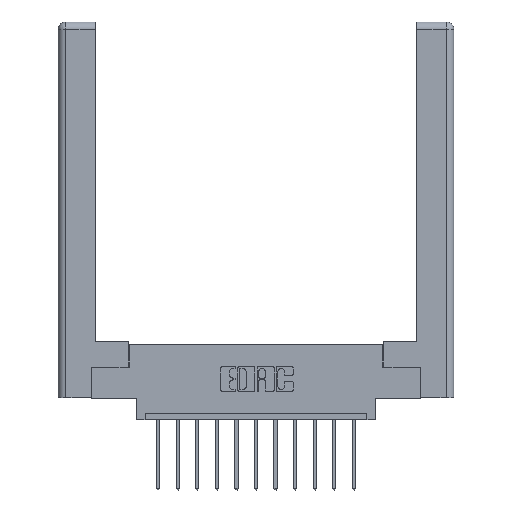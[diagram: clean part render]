
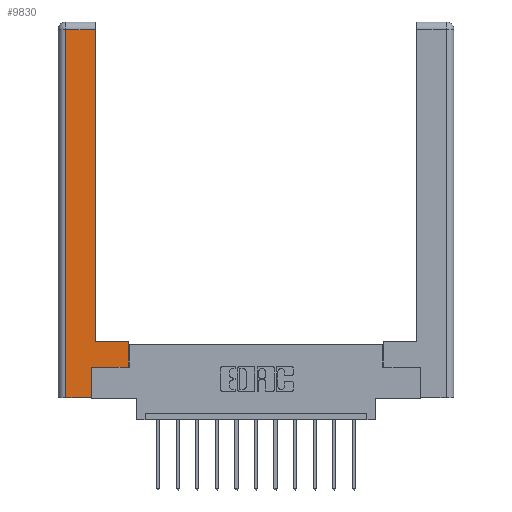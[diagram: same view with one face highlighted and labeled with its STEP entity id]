
A CAD part, top view. The second image highlights one B-rep face of the part: STEP entity #9830.
In plain terms, the highlighted planar face has unit normal (0, 0, 1).
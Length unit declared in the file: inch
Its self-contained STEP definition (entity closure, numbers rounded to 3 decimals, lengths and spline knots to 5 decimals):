
#42 = ORIENTED_EDGE ( 'NONE', *, *, #12930, .T. ) ;
#120 = ORIENTED_EDGE ( 'NONE', *, *, #3742, .T. ) ;
#943 = EDGE_LOOP ( 'NONE', ( #3057, #42, #7764, #14401, #6972, #7880, #6379, #120 ) ) ;
#1010 = CARTESIAN_POINT ( 'NONE',  ( 0., 0., 0. ) ) ;
#1068 = DIRECTION ( 'NONE',  ( -1., 0., 0. ) ) ;
#1400 = EDGE_CURVE ( 'NONE', #2829, #3578, #2583, .T. ) ;
#1668 = VECTOR ( 'NONE', #1682, 39.37008 ) ;
#1682 = DIRECTION ( 'NONE',  ( 0., 1., 0. ) ) ;
#1726 = CARTESIAN_POINT ( 'NONE',  ( 0.295, 0.45, 0. ) ) ;
#2386 = CARTESIAN_POINT ( 'NONE',  ( 0.295, 2.94, 0. ) ) ;
#2583 = LINE ( 'NONE', #3618, #6916 ) ;
#2677 = FACE_OUTER_BOUND ( 'NONE', #943, .T. ) ;
#2763 = DIRECTION ( 'NONE',  ( 1., 0., 0. ) ) ;
#2829 = VERTEX_POINT ( 'NONE', #6642 ) ;
#2945 = EDGE_CURVE ( 'NONE', #5916, #13900, #9573, .T. ) ;
#3057 = ORIENTED_EDGE ( 'NONE', *, *, #3070, .T. ) ;
#3070 = EDGE_CURVE ( 'NONE', #6161, #14623, #10850, .T. ) ;
#3214 = CARTESIAN_POINT ( 'NONE',  ( 0.265, 0.245, 0. ) ) ;
#3449 = CARTESIAN_POINT ( 'NONE',  ( 0.0615, 2.94, 0. ) ) ;
#3578 = VERTEX_POINT ( 'NONE', #8642 ) ;
#3618 = CARTESIAN_POINT ( 'NONE',  ( 0.0615, 0., 0. ) ) ;
#3707 = CARTESIAN_POINT ( 'NONE',  ( 0.565, 0.245, 0. ) ) ;
#3742 = EDGE_CURVE ( 'NONE', #14332, #6161, #13538, .T. ) ;
#3994 = CARTESIAN_POINT ( 'NONE',  ( 0.565, 0.45, 0. ) ) ;
#4100 = VECTOR ( 'NONE', #7072, 39.37008 ) ;
#4303 = CARTESIAN_POINT ( 'NONE',  ( 0.565, 0.245, 0. ) ) ;
#4355 = EDGE_CURVE ( 'NONE', #11036, #5916, #10983, .T. ) ;
#4545 = CARTESIAN_POINT ( 'NONE',  ( 0.295, 0.45, 0. ) ) ;
#4731 = LINE ( 'NONE', #9808, #1668 ) ;
#5916 = VERTEX_POINT ( 'NONE', #3214 ) ;
#5958 = CARTESIAN_POINT ( 'NONE',  ( 0.265, 0.245, 0. ) ) ;
#6161 = VERTEX_POINT ( 'NONE', #1726 ) ;
#6379 = ORIENTED_EDGE ( 'NONE', *, *, #6907, .T. ) ;
#6642 = CARTESIAN_POINT ( 'NONE',  ( 0.0615, 2.94, 0. ) ) ;
#6737 = EDGE_CURVE ( 'NONE', #3578, #11036, #13072, .T. ) ;
#6907 = EDGE_CURVE ( 'NONE', #13900, #14332, #4731, .T. ) ;
#6916 = VECTOR ( 'NONE', #13953, 39.37008 ) ;
#6972 = ORIENTED_EDGE ( 'NONE', *, *, #4355, .T. ) ;
#7009 = LINE ( 'NONE', #3449, #7558 ) ;
#7019 = AXIS2_PLACEMENT_3D ( 'NONE', #1010, #14952, #1068 ) ;
#7072 = DIRECTION ( 'NONE',  ( 0., 1., 0. ) ) ;
#7558 = VECTOR ( 'NONE', #12608, 39.37008 ) ;
#7645 = DIRECTION ( 'NONE',  ( 0., 1., 0. ) ) ;
#7764 = ORIENTED_EDGE ( 'NONE', *, *, #1400, .T. ) ;
#7880 = ORIENTED_EDGE ( 'NONE', *, *, #2945, .T. ) ;
#8537 = CARTESIAN_POINT ( 'NONE',  ( 0.265, 0., 0. ) ) ;
#8642 = CARTESIAN_POINT ( 'NONE',  ( 0.0615, 0., 0. ) ) ;
#8945 = DIRECTION ( 'NONE',  ( -1., 0., 0. ) ) ;
#9573 = LINE ( 'NONE', #3707, #11774 ) ;
#9808 = CARTESIAN_POINT ( 'NONE',  ( 0.565, 0.45, 0. ) ) ;
#9830 = ADVANCED_FACE ( 'NONE', ( #2677 ), #10361, .F. ) ;
#10141 = VECTOR ( 'NONE', #7645, 39.37008 ) ;
#10361 = PLANE ( 'NONE',  #7019 ) ;
#10648 = VECTOR ( 'NONE', #8945, 39.37008 ) ;
#10850 = LINE ( 'NONE', #11187, #10141 ) ;
#10983 = LINE ( 'NONE', #5958, #4100 ) ;
#11036 = VERTEX_POINT ( 'NONE', #12662 ) ;
#11085 = VECTOR ( 'NONE', #2763, 39.37008 ) ;
#11187 = CARTESIAN_POINT ( 'NONE',  ( 0.295, 3., 0. ) ) ;
#11774 = VECTOR ( 'NONE', #11822, 39.37008 ) ;
#11822 = DIRECTION ( 'NONE',  ( 1., 0., 0. ) ) ;
#12608 = DIRECTION ( 'NONE',  ( -1., 0., 0. ) ) ;
#12662 = CARTESIAN_POINT ( 'NONE',  ( 0.265, 0., 0. ) ) ;
#12930 = EDGE_CURVE ( 'NONE', #14623, #2829, #7009, .T. ) ;
#13072 = LINE ( 'NONE', #8537, #11085 ) ;
#13538 = LINE ( 'NONE', #4545, #10648 ) ;
#13900 = VERTEX_POINT ( 'NONE', #4303 ) ;
#13953 = DIRECTION ( 'NONE',  ( 0., -1., 0. ) ) ;
#14332 = VERTEX_POINT ( 'NONE', #3994 ) ;
#14401 = ORIENTED_EDGE ( 'NONE', *, *, #6737, .T. ) ;
#14623 = VERTEX_POINT ( 'NONE', #2386 ) ;
#14952 = DIRECTION ( 'NONE',  ( 0., 0., -1. ) ) ;
